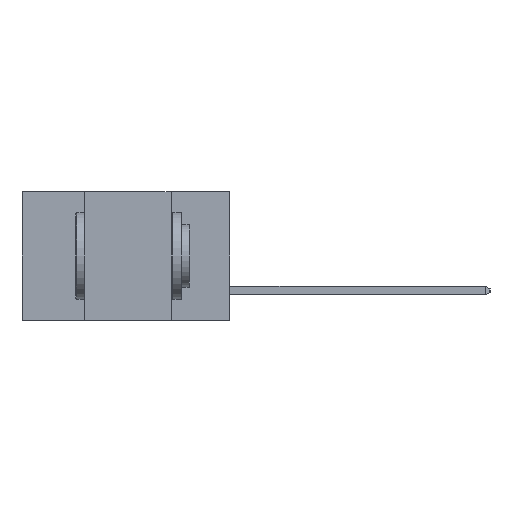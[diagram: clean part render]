
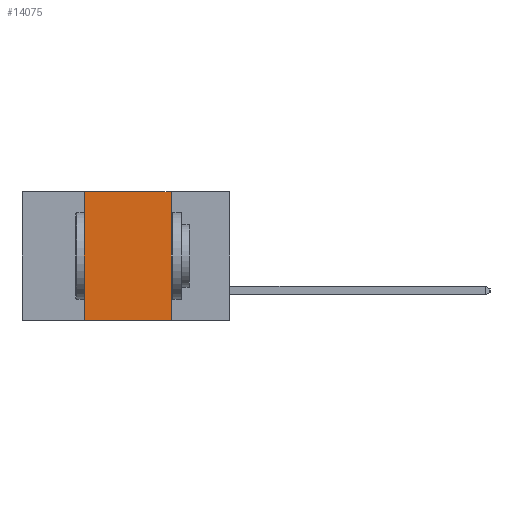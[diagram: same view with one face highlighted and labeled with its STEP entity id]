
A CAD part, left-side view. The second image highlights one B-rep face of the part: STEP entity #14075.
In plain terms, the highlighted planar face has unit normal (-1, 0, 0).
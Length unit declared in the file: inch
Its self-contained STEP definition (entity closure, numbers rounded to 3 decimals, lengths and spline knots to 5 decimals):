
#99 = DIRECTION ( 'NONE',  ( 0., -1., 0. ) ) ;
#649 = EDGE_CURVE ( 'NONE', #12542, #7200, #6282, .T. ) ;
#1509 = EDGE_CURVE ( 'NONE', #4490, #12192, #5150, .T. ) ;
#2227 = ORIENTED_EDGE ( 'NONE', *, *, #1509, .F. ) ;
#2269 = CARTESIAN_POINT ( 'NONE',  ( 0., 0.6, 0. ) ) ;
#2382 = EDGE_CURVE ( 'NONE', #4490, #7200, #9864, .T. ) ;
#2411 = LINE ( 'NONE', #9628, #7671 ) ;
#2892 = DIRECTION ( 'NONE',  ( 0., -1., 0. ) ) ;
#2919 = CARTESIAN_POINT ( 'NONE',  ( 0., 0.6, -0.37 ) ) ;
#3125 = EDGE_CURVE ( 'NONE', #12192, #12542, #2411, .T. ) ;
#3524 = DIRECTION ( 'NONE',  ( 0., 0., -1. ) ) ;
#4490 = VERTEX_POINT ( 'NONE', #4781 ) ;
#4781 = CARTESIAN_POINT ( 'NONE',  ( 0., 0.42, -0.37 ) ) ;
#5141 = ORIENTED_EDGE ( 'NONE', *, *, #3125, .F. ) ;
#5150 = LINE ( 'NONE', #13739, #10988 ) ;
#5511 = ORIENTED_EDGE ( 'NONE', *, *, #2382, .T. ) ;
#6282 = LINE ( 'NONE', #8062, #14671 ) ;
#7200 = VERTEX_POINT ( 'NONE', #12106 ) ;
#7671 = VECTOR ( 'NONE', #99, 39.37008 ) ;
#8062 = CARTESIAN_POINT ( 'NONE',  ( 0., 0.17, 0. ) ) ;
#8064 = CARTESIAN_POINT ( 'NONE',  ( 0., 0.17, 0. ) ) ;
#8249 = FACE_OUTER_BOUND ( 'NONE', #9208, .T. ) ;
#9208 = EDGE_LOOP ( 'NONE', ( #13993, #5141, #2227, #5511 ) ) ;
#9418 = PLANE ( 'NONE',  #9710 ) ;
#9628 = CARTESIAN_POINT ( 'NONE',  ( 0., 0.6, 0. ) ) ;
#9710 = AXIS2_PLACEMENT_3D ( 'NONE', #2269, #10588, #3524 ) ;
#9726 = DIRECTION ( 'NONE',  ( 0., 0., -1. ) ) ;
#9746 = CARTESIAN_POINT ( 'NONE',  ( 0., 0.42, 0. ) ) ;
#9864 = LINE ( 'NONE', #2919, #12563 ) ;
#10588 = DIRECTION ( 'NONE',  ( 1., 0., 0. ) ) ;
#10988 = VECTOR ( 'NONE', #13697, 39.37008 ) ;
#12106 = CARTESIAN_POINT ( 'NONE',  ( 0., 0.17, -0.37 ) ) ;
#12192 = VERTEX_POINT ( 'NONE', #9746 ) ;
#12542 = VERTEX_POINT ( 'NONE', #8064 ) ;
#12563 = VECTOR ( 'NONE', #2892, 39.37008 ) ;
#13697 = DIRECTION ( 'NONE',  ( 0., 0., 1. ) ) ;
#13739 = CARTESIAN_POINT ( 'NONE',  ( 0., 0.42, 0. ) ) ;
#13993 = ORIENTED_EDGE ( 'NONE', *, *, #649, .F. ) ;
#14075 = ADVANCED_FACE ( 'NONE', ( #8249 ), #9418, .F. ) ;
#14671 = VECTOR ( 'NONE', #9726, 39.37008 ) ;
